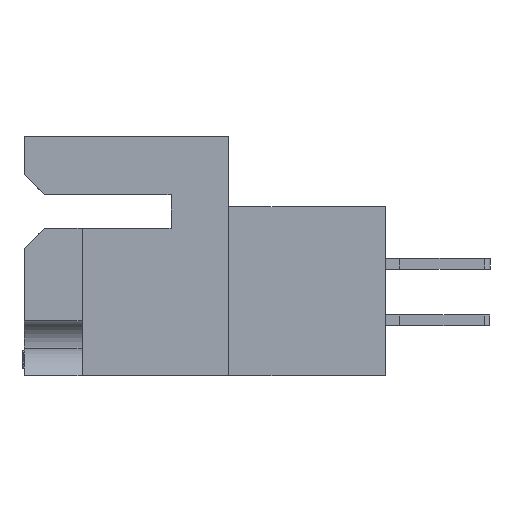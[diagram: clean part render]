
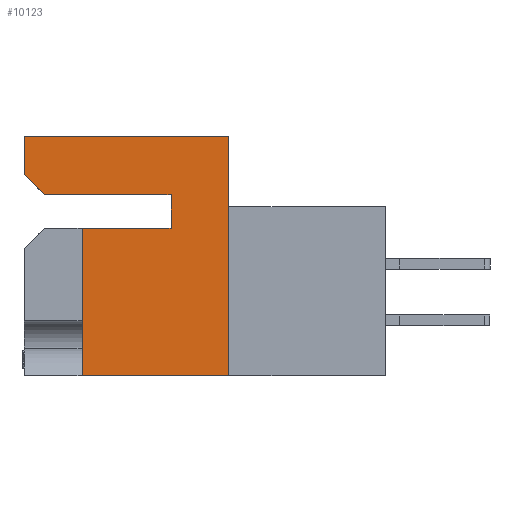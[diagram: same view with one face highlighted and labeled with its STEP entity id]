
A CAD part, left-side view. The second image highlights one B-rep face of the part: STEP entity #10123.
In plain terms, the highlighted planar face has unit normal (-1, 0, 0).
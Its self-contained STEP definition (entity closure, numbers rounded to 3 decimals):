
#70 = CARTESIAN_POINT ( 'NONE',  ( 0., 8.255, -13.487 ) ) ;
#257 = DIRECTION ( 'NONE',  ( 0., 0., 1. ) ) ;
#944 = CARTESIAN_POINT ( 'NONE',  ( 0., 11.506, 0. ) ) ;
#1108 = VECTOR ( 'NONE', #17500, 1000. ) ;
#1334 = EDGE_CURVE ( 'NONE', #3580, #15113, #15296, .T. ) ;
#1413 = VERTEX_POINT ( 'NONE', #13499 ) ;
#1488 = LINE ( 'NONE', #15026, #2954 ) ;
#1714 = VECTOR ( 'NONE', #4568, 1000. ) ;
#1951 = EDGE_CURVE ( 'NONE', #4620, #9934, #23767, .T. ) ;
#2029 = LINE ( 'NONE', #13834, #1714 ) ;
#2320 = EDGE_CURVE ( 'NONE', #9934, #1413, #4103, .T. ) ;
#2386 = VECTOR ( 'NONE', #7103, 1000. ) ;
#2954 = VECTOR ( 'NONE', #20585, 1000. ) ;
#3580 = VERTEX_POINT ( 'NONE', #944 ) ;
#3758 = CARTESIAN_POINT ( 'NONE',  ( 0., 11.506, 0. ) ) ;
#3814 = ORIENTED_EDGE ( 'NONE', *, *, #15802, .F. ) ;
#4103 = LINE ( 'NONE', #23774, #4388 ) ;
#4294 = VECTOR ( 'NONE', #16360, 1000. ) ;
#4388 = VECTOR ( 'NONE', #16264, 1000. ) ;
#4407 = PLANE ( 'NONE',  #17089 ) ;
#4568 = DIRECTION ( 'NONE',  ( 0., -1., 0. ) ) ;
#4620 = VERTEX_POINT ( 'NONE', #6076 ) ;
#4892 = CARTESIAN_POINT ( 'NONE',  ( 0., 0., 0. ) ) ;
#4929 = FACE_OUTER_BOUND ( 'NONE', #8468, .T. ) ;
#5020 = CARTESIAN_POINT ( 'NONE',  ( 0., 0., 0. ) ) ;
#5457 = LINE ( 'NONE', #5020, #4294 ) ;
#5514 = ORIENTED_EDGE ( 'NONE', *, *, #10117, .F. ) ;
#6076 = CARTESIAN_POINT ( 'NONE',  ( 0., 0., -13.487 ) ) ;
#6120 = DIRECTION ( 'NONE',  ( 0., 1., 0. ) ) ;
#6194 = DIRECTION ( 'NONE',  ( 0., 0., -1. ) ) ;
#6383 = LINE ( 'NONE', #11490, #16968 ) ;
#6898 = VERTEX_POINT ( 'NONE', #13192 ) ;
#7103 = DIRECTION ( 'NONE',  ( 0., -1., 0. ) ) ;
#7636 = VECTOR ( 'NONE', #24114, 1000. ) ;
#8341 = DIRECTION ( 'NONE',  ( 1., 0., 0. ) ) ;
#8468 = EDGE_LOOP ( 'NONE', ( #11598, #20711, #9749, #14283, #20908, #17572, #3814, #5514, #20595 ) ) ;
#9749 = ORIENTED_EDGE ( 'NONE', *, *, #1334, .F. ) ;
#9888 = VECTOR ( 'NONE', #6120, 1000. ) ;
#9934 = VERTEX_POINT ( 'NONE', #70 ) ;
#10117 = EDGE_CURVE ( 'NONE', #1413, #6898, #2029, .T. ) ;
#10123 = ADVANCED_FACE ( 'NONE', ( #4929 ), #4407, .F. ) ;
#10870 = EDGE_CURVE ( 'NONE', #23046, #19937, #14886, .T. ) ;
#11017 = EDGE_CURVE ( 'NONE', #12877, #3580, #22518, .T. ) ;
#11490 = CARTESIAN_POINT ( 'NONE',  ( 0., 3.251, -5.182 ) ) ;
#11598 = ORIENTED_EDGE ( 'NONE', *, *, #1951, .F. ) ;
#12877 = VERTEX_POINT ( 'NONE', #13566 ) ;
#12996 = CARTESIAN_POINT ( 'NONE',  ( 0., 10.363, -3.302 ) ) ;
#13192 = CARTESIAN_POINT ( 'NONE',  ( 0., 3.251, -5.182 ) ) ;
#13499 = CARTESIAN_POINT ( 'NONE',  ( 0., 8.255, -5.182 ) ) ;
#13566 = CARTESIAN_POINT ( 'NONE',  ( 0., 11.506, -2.159 ) ) ;
#13699 = CARTESIAN_POINT ( 'NONE',  ( 0., 3.251, -3.302 ) ) ;
#13834 = CARTESIAN_POINT ( 'NONE',  ( 0., 0., -5.182 ) ) ;
#14283 = ORIENTED_EDGE ( 'NONE', *, *, #11017, .F. ) ;
#14792 = CARTESIAN_POINT ( 'NONE',  ( 0., -8.814, -13.487 ) ) ;
#14866 = EDGE_CURVE ( 'NONE', #12877, #19937, #1488, .T. ) ;
#14886 = LINE ( 'NONE', #15409, #9888 ) ;
#15026 = CARTESIAN_POINT ( 'NONE',  ( 0., 10.363, -3.302 ) ) ;
#15113 = VERTEX_POINT ( 'NONE', #4892 ) ;
#15296 = LINE ( 'NONE', #3758, #2386 ) ;
#15409 = CARTESIAN_POINT ( 'NONE',  ( 0., 0., -3.302 ) ) ;
#15516 = CARTESIAN_POINT ( 'NONE',  ( 0., 11.506, -13.487 ) ) ;
#15802 = EDGE_CURVE ( 'NONE', #6898, #23046, #6383, .T. ) ;
#16264 = DIRECTION ( 'NONE',  ( 0., 0., 1. ) ) ;
#16360 = DIRECTION ( 'NONE',  ( 0., 0., -1. ) ) ;
#16968 = VECTOR ( 'NONE', #257, 1000. ) ;
#17089 = AXIS2_PLACEMENT_3D ( 'NONE', #19572, #8341, #6194 ) ;
#17500 = DIRECTION ( 'NONE',  ( 0., 0., 1. ) ) ;
#17572 = ORIENTED_EDGE ( 'NONE', *, *, #10870, .F. ) ;
#17787 = EDGE_CURVE ( 'NONE', #15113, #4620, #5457, .T. ) ;
#19572 = CARTESIAN_POINT ( 'NONE',  ( 0., 0., 0. ) ) ;
#19937 = VERTEX_POINT ( 'NONE', #12996 ) ;
#20585 = DIRECTION ( 'NONE',  ( 0., -0.707, -0.707 ) ) ;
#20595 = ORIENTED_EDGE ( 'NONE', *, *, #2320, .F. ) ;
#20711 = ORIENTED_EDGE ( 'NONE', *, *, #17787, .F. ) ;
#20908 = ORIENTED_EDGE ( 'NONE', *, *, #14866, .T. ) ;
#22518 = LINE ( 'NONE', #15516, #1108 ) ;
#23046 = VERTEX_POINT ( 'NONE', #13699 ) ;
#23767 = LINE ( 'NONE', #14792, #7636 ) ;
#23774 = CARTESIAN_POINT ( 'NONE',  ( 0., 8.255, -5.182 ) ) ;
#24114 = DIRECTION ( 'NONE',  ( 0., 1., 0. ) ) ;
